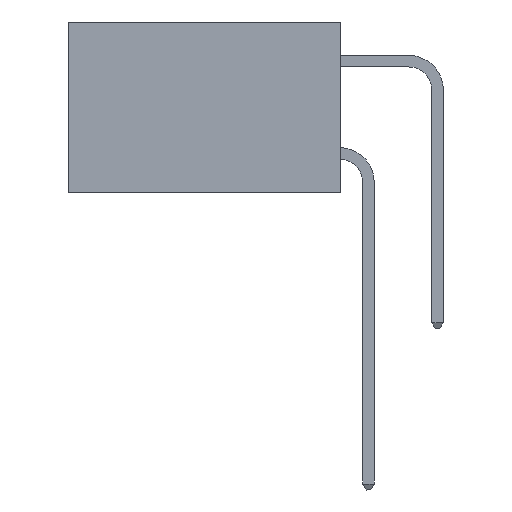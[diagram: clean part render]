
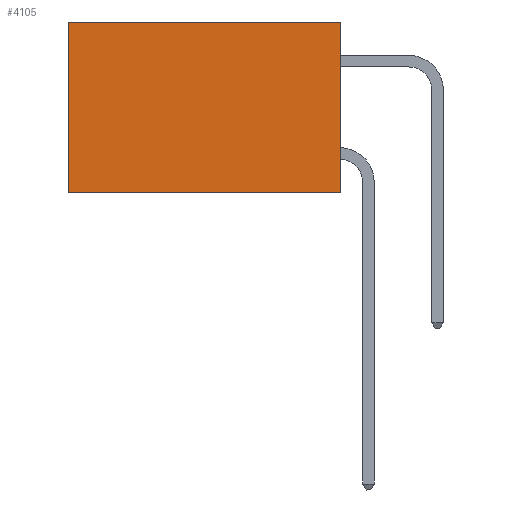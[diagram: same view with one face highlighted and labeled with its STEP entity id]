
A CAD part, left-side view. The second image highlights one B-rep face of the part: STEP entity #4105.
In plain terms, the highlighted planar face has unit normal (-1, 0, 0).
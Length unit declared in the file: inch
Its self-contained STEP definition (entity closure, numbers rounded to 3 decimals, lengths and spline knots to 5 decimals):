
#558 = VECTOR ( 'NONE', #10139, 39.37008 ) ;
#668 = EDGE_LOOP ( 'NONE', ( #10189, #4040, #6767, #4638 ) ) ;
#1195 = AXIS2_PLACEMENT_3D ( 'NONE', #8454, #8647, #8248 ) ;
#2382 = DIRECTION ( 'NONE',  ( 0., 0., -1. ) ) ;
#2484 = CARTESIAN_POINT ( 'NONE',  ( 0.277, 0.59, -0.37 ) ) ;
#3354 = VERTEX_POINT ( 'NONE', #11776 ) ;
#3535 = EDGE_CURVE ( 'NONE', #6412, #4448, #5471, .T. ) ;
#3588 = EDGE_CURVE ( 'NONE', #3354, #9124, #6698, .T. ) ;
#3611 = CARTESIAN_POINT ( 'NONE',  ( 0.277, 0.59, 0. ) ) ;
#3613 = EDGE_CURVE ( 'NONE', #3354, #6412, #6430, .T. ) ;
#3699 = CARTESIAN_POINT ( 'NONE',  ( 0.277, 0., -0.37 ) ) ;
#3873 = EDGE_CURVE ( 'NONE', #9124, #4448, #8356, .T. ) ;
#3936 = FACE_OUTER_BOUND ( 'NONE', #668, .T. ) ;
#4040 = ORIENTED_EDGE ( 'NONE', *, *, #3535, .F. ) ;
#4105 = ADVANCED_FACE ( 'NONE', ( #3936 ), #8312, .F. ) ;
#4448 = VERTEX_POINT ( 'NONE', #11616 ) ;
#4638 = ORIENTED_EDGE ( 'NONE', *, *, #3588, .T. ) ;
#5471 = LINE ( 'NONE', #5814, #9731 ) ;
#5814 = CARTESIAN_POINT ( 'NONE',  ( 0.277, 0., -0.37 ) ) ;
#5895 = VECTOR ( 'NONE', #2382, 39.37008 ) ;
#5977 = DIRECTION ( 'NONE',  ( 0., 1., 0. ) ) ;
#6412 = VERTEX_POINT ( 'NONE', #3699 ) ;
#6430 = LINE ( 'NONE', #10250, #558 ) ;
#6698 = LINE ( 'NONE', #10779, #10640 ) ;
#6767 = ORIENTED_EDGE ( 'NONE', *, *, #3613, .F. ) ;
#8248 = DIRECTION ( 'NONE',  ( 0., 0., -1. ) ) ;
#8312 = PLANE ( 'NONE',  #1195 ) ;
#8356 = LINE ( 'NONE', #2484, #5895 ) ;
#8454 = CARTESIAN_POINT ( 'NONE',  ( 0.277, 0., -0.37 ) ) ;
#8647 = DIRECTION ( 'NONE',  ( 1., 0., 0. ) ) ;
#9124 = VERTEX_POINT ( 'NONE', #3611 ) ;
#9731 = VECTOR ( 'NONE', #5977, 39.37008 ) ;
#10139 = DIRECTION ( 'NONE',  ( 0., 0., -1. ) ) ;
#10189 = ORIENTED_EDGE ( 'NONE', *, *, #3873, .T. ) ;
#10250 = CARTESIAN_POINT ( 'NONE',  ( 0.277, 0., -0.37 ) ) ;
#10640 = VECTOR ( 'NONE', #10790, 39.37008 ) ;
#10779 = CARTESIAN_POINT ( 'NONE',  ( 0.277, 0., 0. ) ) ;
#10790 = DIRECTION ( 'NONE',  ( 0., 1., 0. ) ) ;
#11616 = CARTESIAN_POINT ( 'NONE',  ( 0.277, 0.59, -0.37 ) ) ;
#11776 = CARTESIAN_POINT ( 'NONE',  ( 0.277, 0., 0. ) ) ;
